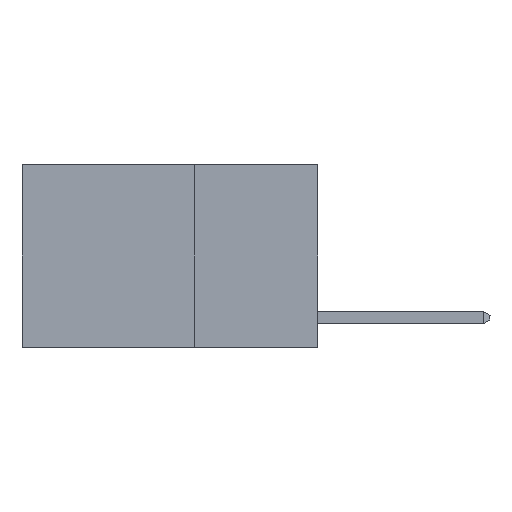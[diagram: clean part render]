
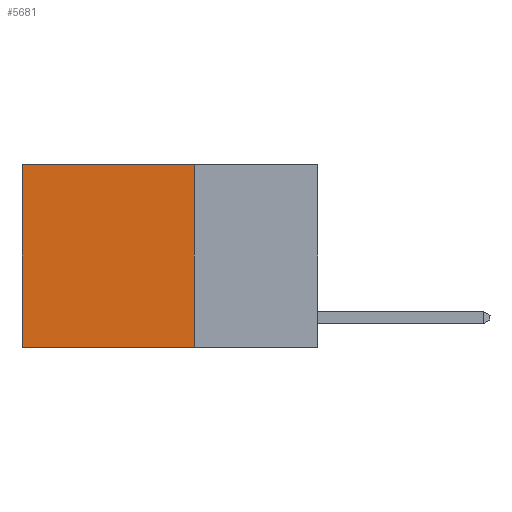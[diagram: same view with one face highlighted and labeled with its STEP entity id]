
A CAD part, left-side view. The second image highlights one B-rep face of the part: STEP entity #5681.
In plain terms, the highlighted planar face has unit normal (-1, 0, 0).
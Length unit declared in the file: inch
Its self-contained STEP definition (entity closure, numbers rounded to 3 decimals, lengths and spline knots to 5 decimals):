
#170 = CARTESIAN_POINT ( 'NONE',  ( 0.2625, 0.6, 0. ) ) ;
#298 = CARTESIAN_POINT ( 'NONE',  ( 0.2625, 0.6, -0.37 ) ) ;
#671 = DIRECTION ( 'NONE',  ( 0., 1., 0. ) ) ;
#1302 = CARTESIAN_POINT ( 'NONE',  ( 0.2625, 0.25, 0. ) ) ;
#1400 = ORIENTED_EDGE ( 'NONE', *, *, #3696, .F. ) ;
#1886 = VERTEX_POINT ( 'NONE', #6338 ) ;
#2084 = VECTOR ( 'NONE', #671, 39.37008 ) ;
#2149 = LINE ( 'NONE', #170, #5231 ) ;
#2684 = VECTOR ( 'NONE', #3911, 39.37008 ) ;
#2696 = LINE ( 'NONE', #8037, #2084 ) ;
#3330 = CARTESIAN_POINT ( 'NONE',  ( 0.2625, 0.25, 0. ) ) ;
#3696 = EDGE_CURVE ( 'NONE', #5990, #1886, #5470, .T. ) ;
#3911 = DIRECTION ( 'NONE',  ( 0., 1., 0. ) ) ;
#3999 = VERTEX_POINT ( 'NONE', #298 ) ;
#4150 = CARTESIAN_POINT ( 'NONE',  ( 0.2625, 0.25, 0. ) ) ;
#4419 = AXIS2_PLACEMENT_3D ( 'NONE', #4150, #6587, #5385 ) ;
#4626 = LINE ( 'NONE', #3330, #2684 ) ;
#4692 = ORIENTED_EDGE ( 'NONE', *, *, #5182, .F. ) ;
#4792 = EDGE_LOOP ( 'NONE', ( #6883, #4692, #1400, #5896 ) ) ;
#5098 = VERTEX_POINT ( 'NONE', #5388 ) ;
#5099 = EDGE_CURVE ( 'NONE', #5098, #3999, #2149, .T. ) ;
#5182 = EDGE_CURVE ( 'NONE', #1886, #3999, #2696, .T. ) ;
#5228 = VECTOR ( 'NONE', #6750, 39.37008 ) ;
#5231 = VECTOR ( 'NONE', #7391, 39.37008 ) ;
#5264 = PLANE ( 'NONE',  #4419 ) ;
#5385 = DIRECTION ( 'NONE',  ( 0., 0., -1. ) ) ;
#5388 = CARTESIAN_POINT ( 'NONE',  ( 0.2625, 0.6, 0. ) ) ;
#5470 = LINE ( 'NONE', #7411, #5228 ) ;
#5681 = ADVANCED_FACE ( 'NONE', ( #7339 ), #5264, .F. ) ;
#5896 = ORIENTED_EDGE ( 'NONE', *, *, #7260, .T. ) ;
#5990 = VERTEX_POINT ( 'NONE', #1302 ) ;
#6338 = CARTESIAN_POINT ( 'NONE',  ( 0.2625, 0.25, -0.37 ) ) ;
#6587 = DIRECTION ( 'NONE',  ( 1., 0., 0. ) ) ;
#6750 = DIRECTION ( 'NONE',  ( 0., 0., -1. ) ) ;
#6883 = ORIENTED_EDGE ( 'NONE', *, *, #5099, .T. ) ;
#7260 = EDGE_CURVE ( 'NONE', #5990, #5098, #4626, .T. ) ;
#7339 = FACE_OUTER_BOUND ( 'NONE', #4792, .T. ) ;
#7391 = DIRECTION ( 'NONE',  ( 0., 0., -1. ) ) ;
#7411 = CARTESIAN_POINT ( 'NONE',  ( 0.2625, 0.25, 0. ) ) ;
#8037 = CARTESIAN_POINT ( 'NONE',  ( 0.2625, 0.25, -0.37 ) ) ;
